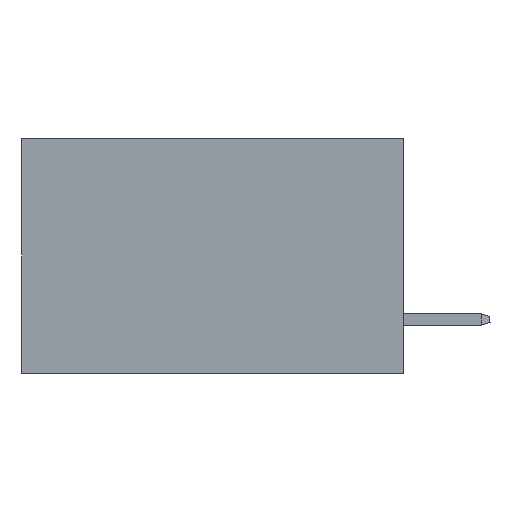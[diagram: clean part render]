
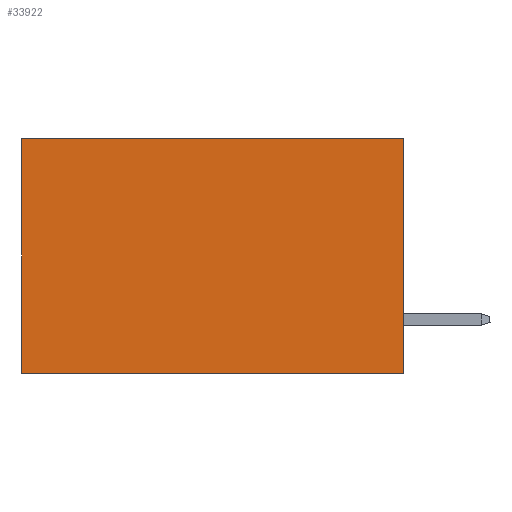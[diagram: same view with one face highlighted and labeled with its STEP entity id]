
A CAD part, left-side view. The second image highlights one B-rep face of the part: STEP entity #33922.
In plain terms, the highlighted planar face has unit normal (-1, 0, 0).
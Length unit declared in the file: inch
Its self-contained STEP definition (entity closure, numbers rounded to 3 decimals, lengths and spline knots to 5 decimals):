
#544 = ORIENTED_EDGE ( 'NONE', *, *, #31912, .T. ) ;
#3397 = EDGE_CURVE ( 'NONE', #6909, #35171, #11857, .T. ) ;
#4600 = EDGE_CURVE ( 'NONE', #17397, #6909, #36057, .T. ) ;
#5065 = FACE_OUTER_BOUND ( 'NONE', #37214, .T. ) ;
#6909 = VERTEX_POINT ( 'NONE', #37316 ) ;
#7123 = CARTESIAN_POINT ( 'NONE',  ( 0.2875, 0.6, 0. ) ) ;
#8223 = CARTESIAN_POINT ( 'NONE',  ( 0.2875, 0.6, 0. ) ) ;
#9385 = VECTOR ( 'NONE', #26791, 39.37008 ) ;
#10518 = CARTESIAN_POINT ( 'NONE',  ( 0.2875, 0., 0. ) ) ;
#11857 = LINE ( 'NONE', #36892, #9385 ) ;
#12286 = PLANE ( 'NONE',  #31267 ) ;
#13947 = VECTOR ( 'NONE', #25007, 39.37008 ) ;
#14139 = CARTESIAN_POINT ( 'NONE',  ( 0.2875, 0., 0. ) ) ;
#17397 = VERTEX_POINT ( 'NONE', #14139 ) ;
#18256 = CARTESIAN_POINT ( 'NONE',  ( 0.2875, 0., 0. ) ) ;
#18513 = LINE ( 'NONE', #8223, #24152 ) ;
#18779 = ORIENTED_EDGE ( 'NONE', *, *, #26942, .T. ) ;
#21507 = LINE ( 'NONE', #10518, #13947 ) ;
#23733 = CARTESIAN_POINT ( 'NONE',  ( 0.2875, 0., 0. ) ) ;
#23787 = VERTEX_POINT ( 'NONE', #7123 ) ;
#24152 = VECTOR ( 'NONE', #36981, 39.37008 ) ;
#24334 = ORIENTED_EDGE ( 'NONE', *, *, #3397, .F. ) ;
#25007 = DIRECTION ( 'NONE',  ( 0., 1., 0. ) ) ;
#26791 = DIRECTION ( 'NONE',  ( 0., 1., 0. ) ) ;
#26942 = EDGE_CURVE ( 'NONE', #23787, #35171, #18513, .T. ) ;
#28566 = DIRECTION ( 'NONE',  ( 0., 0., -1. ) ) ;
#30548 = DIRECTION ( 'NONE',  ( 0., 0., -1. ) ) ;
#31267 = AXIS2_PLACEMENT_3D ( 'NONE', #23733, #45049, #30548 ) ;
#31912 = EDGE_CURVE ( 'NONE', #17397, #23787, #21507, .T. ) ;
#33922 = ADVANCED_FACE ( 'NONE', ( #5065 ), #12286, .F. ) ;
#35171 = VERTEX_POINT ( 'NONE', #45059 ) ;
#36057 = LINE ( 'NONE', #18256, #41339 ) ;
#36892 = CARTESIAN_POINT ( 'NONE',  ( 0.2875, 0., -0.37 ) ) ;
#36981 = DIRECTION ( 'NONE',  ( 0., 0., -1. ) ) ;
#37214 = EDGE_LOOP ( 'NONE', ( #18779, #24334, #45885, #544 ) ) ;
#37316 = CARTESIAN_POINT ( 'NONE',  ( 0.2875, 0., -0.37 ) ) ;
#41339 = VECTOR ( 'NONE', #28566, 39.37008 ) ;
#45049 = DIRECTION ( 'NONE',  ( 1., 0., 0. ) ) ;
#45059 = CARTESIAN_POINT ( 'NONE',  ( 0.2875, 0.6, -0.37 ) ) ;
#45885 = ORIENTED_EDGE ( 'NONE', *, *, #4600, .F. ) ;
